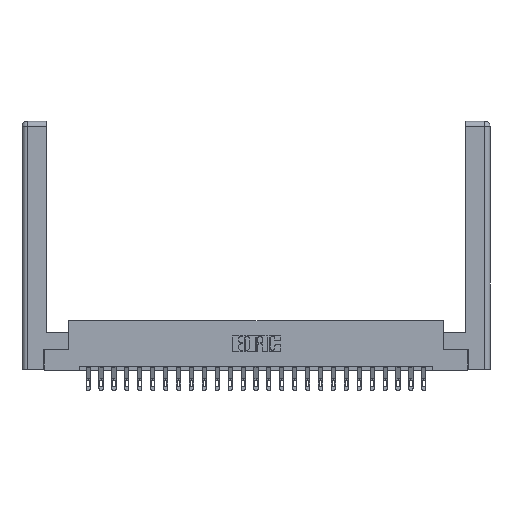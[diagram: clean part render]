
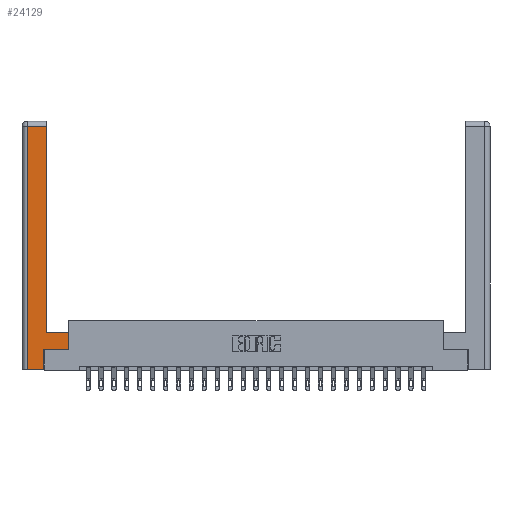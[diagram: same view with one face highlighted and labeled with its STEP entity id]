
A CAD part, top view. The second image highlights one B-rep face of the part: STEP entity #24129.
In plain terms, the highlighted planar face has unit normal (0, 0, 1).
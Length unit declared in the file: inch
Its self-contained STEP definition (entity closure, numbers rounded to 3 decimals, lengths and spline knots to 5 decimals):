
#618 = EDGE_CURVE ( 'NONE', #25103, #6055, #3236, .T. ) ;
#1242 = VECTOR ( 'NONE', #3392, 39.37008 ) ;
#2244 = CARTESIAN_POINT ( 'NONE',  ( 0.265, 0., 0. ) ) ;
#2901 = ORIENTED_EDGE ( 'NONE', *, *, #9109, .T. ) ;
#3236 = LINE ( 'NONE', #19730, #11985 ) ;
#3294 = LINE ( 'NONE', #2244, #20210 ) ;
#3392 = DIRECTION ( 'NONE',  ( 0., -1., 0. ) ) ;
#3585 = EDGE_CURVE ( 'NONE', #6560, #8295, #23424, .T. ) ;
#3725 = CARTESIAN_POINT ( 'NONE',  ( 0.265, 0.245, 0. ) ) ;
#3736 = EDGE_CURVE ( 'NONE', #13465, #8968, #8722, .T. ) ;
#4017 = CARTESIAN_POINT ( 'NONE',  ( 0.295, 2.94, 0. ) ) ;
#6023 = CARTESIAN_POINT ( 'NONE',  ( 0.0615, 2.94, 0. ) ) ;
#6055 = VERTEX_POINT ( 'NONE', #16769 ) ;
#6560 = VERTEX_POINT ( 'NONE', #10782 ) ;
#6778 = LINE ( 'NONE', #13249, #16189 ) ;
#7135 = DIRECTION ( 'NONE',  ( 0., 1., 0. ) ) ;
#7157 = DIRECTION ( 'NONE',  ( 0., 0., -1. ) ) ;
#7538 = ORIENTED_EDGE ( 'NONE', *, *, #21930, .T. ) ;
#7601 = VERTEX_POINT ( 'NONE', #20840 ) ;
#7814 = LINE ( 'NONE', #20875, #18205 ) ;
#8083 = VECTOR ( 'NONE', #7135, 39.37008 ) ;
#8295 = VERTEX_POINT ( 'NONE', #16547 ) ;
#8722 = LINE ( 'NONE', #3725, #8083 ) ;
#8968 = VERTEX_POINT ( 'NONE', #24886 ) ;
#9109 = EDGE_CURVE ( 'NONE', #7601, #25103, #18114, .T. ) ;
#10782 = CARTESIAN_POINT ( 'NONE',  ( 0.0615, 2.94, 0. ) ) ;
#10912 = AXIS2_PLACEMENT_3D ( 'NONE', #25159, #7157, #23113 ) ;
#11206 = PLANE ( 'NONE',  #10912 ) ;
#11358 = CARTESIAN_POINT ( 'NONE',  ( 0.0615, 0., 0. ) ) ;
#11985 = VECTOR ( 'NONE', #21724, 39.37008 ) ;
#13249 = CARTESIAN_POINT ( 'NONE',  ( 0.295, 3., 0. ) ) ;
#13313 = EDGE_CURVE ( 'NONE', #8968, #7601, #7814, .T. ) ;
#13465 = VERTEX_POINT ( 'NONE', #23202 ) ;
#14255 = LINE ( 'NONE', #6023, #15190 ) ;
#14726 = ORIENTED_EDGE ( 'NONE', *, *, #13313, .T. ) ;
#15172 = DIRECTION ( 'NONE',  ( 0., 1., 0. ) ) ;
#15190 = VECTOR ( 'NONE', #16106, 39.37008 ) ;
#15608 = ORIENTED_EDGE ( 'NONE', *, *, #618, .T. ) ;
#16106 = DIRECTION ( 'NONE',  ( -1., 0., 0. ) ) ;
#16189 = VECTOR ( 'NONE', #15172, 39.37008 ) ;
#16547 = CARTESIAN_POINT ( 'NONE',  ( 0.0615, 0., 0. ) ) ;
#16769 = CARTESIAN_POINT ( 'NONE',  ( 0.295, 0.45, 0. ) ) ;
#17186 = ORIENTED_EDGE ( 'NONE', *, *, #23069, .T. ) ;
#17799 = CARTESIAN_POINT ( 'NONE',  ( 0.565, 0.45, 0. ) ) ;
#18114 = LINE ( 'NONE', #17799, #18752 ) ;
#18205 = VECTOR ( 'NONE', #22533, 39.37008 ) ;
#18600 = FACE_OUTER_BOUND ( 'NONE', #19201, .T. ) ;
#18601 = ORIENTED_EDGE ( 'NONE', *, *, #25778, .T. ) ;
#18752 = VECTOR ( 'NONE', #19815, 39.37008 ) ;
#19201 = EDGE_LOOP ( 'NONE', ( #7538, #17186, #24309, #18601, #21374, #14726, #2901, #15608 ) ) ;
#19730 = CARTESIAN_POINT ( 'NONE',  ( 0.295, 0.45, 0. ) ) ;
#19815 = DIRECTION ( 'NONE',  ( 0., 1., 0. ) ) ;
#20210 = VECTOR ( 'NONE', #22295, 39.37008 ) ;
#20311 = CARTESIAN_POINT ( 'NONE',  ( 0.565, 0.45, 0. ) ) ;
#20840 = CARTESIAN_POINT ( 'NONE',  ( 0.565, 0.245, 0. ) ) ;
#20875 = CARTESIAN_POINT ( 'NONE',  ( 0.565, 0.245, 0. ) ) ;
#21374 = ORIENTED_EDGE ( 'NONE', *, *, #3736, .T. ) ;
#21724 = DIRECTION ( 'NONE',  ( -1., 0., 0. ) ) ;
#21930 = EDGE_CURVE ( 'NONE', #6055, #23061, #6778, .T. ) ;
#22295 = DIRECTION ( 'NONE',  ( 1., 0., 0. ) ) ;
#22533 = DIRECTION ( 'NONE',  ( 1., 0., 0. ) ) ;
#23061 = VERTEX_POINT ( 'NONE', #4017 ) ;
#23069 = EDGE_CURVE ( 'NONE', #23061, #6560, #14255, .T. ) ;
#23113 = DIRECTION ( 'NONE',  ( -1., 0., 0. ) ) ;
#23202 = CARTESIAN_POINT ( 'NONE',  ( 0.265, 0., 0. ) ) ;
#23424 = LINE ( 'NONE', #11358, #1242 ) ;
#24129 = ADVANCED_FACE ( 'NONE', ( #18600 ), #11206, .F. ) ;
#24309 = ORIENTED_EDGE ( 'NONE', *, *, #3585, .T. ) ;
#24886 = CARTESIAN_POINT ( 'NONE',  ( 0.265, 0.245, 0. ) ) ;
#25103 = VERTEX_POINT ( 'NONE', #20311 ) ;
#25159 = CARTESIAN_POINT ( 'NONE',  ( 0., 0., 0. ) ) ;
#25778 = EDGE_CURVE ( 'NONE', #8295, #13465, #3294, .T. ) ;
